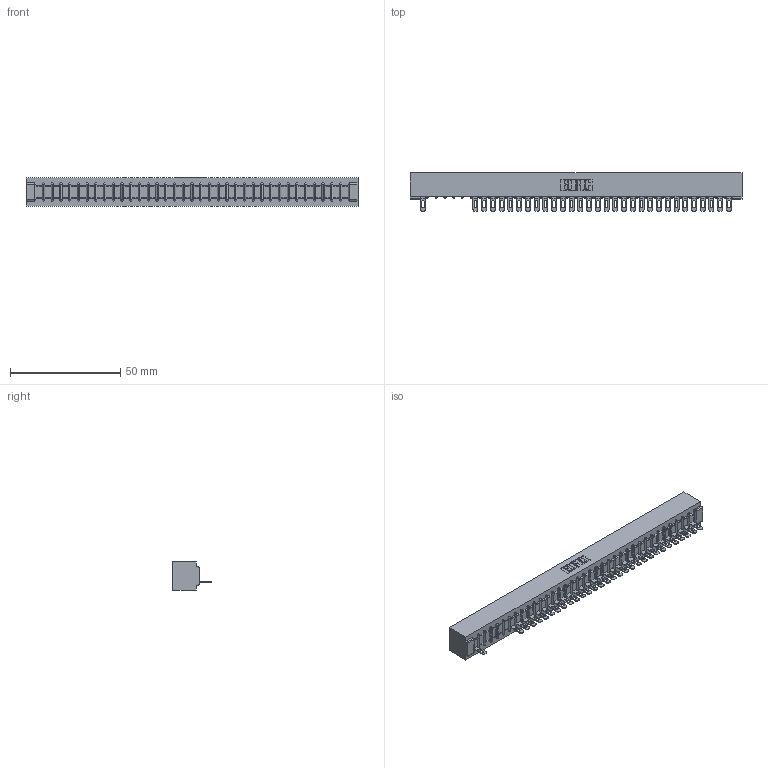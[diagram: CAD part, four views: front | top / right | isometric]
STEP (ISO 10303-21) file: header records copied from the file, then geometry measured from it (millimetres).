
FILE_DESCRIPTION (( 'STEP AP203' ), '1' );
FILE_NAME ('357-036-501-101.STEP', '2018-08-10T05:33:35', ( '' ), ( '' ), 'SwSTEP 2.0', 'SolidWorks 2016', '' );
FILE_SCHEMA (( 'CONFIG_CONTROL_DESIGN' ));
Length unit declared in the file: inch
Products named in the file (3): 307 Part_No Mounting Lugs; 307-290-002_501; 357-036-501-101
Assembly tree (32 placements, depth 2):
  357-036-501-101
    307 Part_No Mounting Lugs
    307-290-002_501  x31
Bounding box: 150.52 x 17.42 x 12.7 mm (x, y, z)
Volume: 16502.9 mm3; surface area: 20251 mm2
Topology: 32 solids, 32 shells, 2603 faces, 7997 edges, 5230 vertices
Faces by surface type: plane 1490, cylinder 1039, sphere 74
Entity records: 31958 total; most frequent: CARTESIAN_POINT 5411, ORIENTED_EDGE 5406, DIRECTION 5257, EDGE_CURVE 2703, VECTOR 2065, LINE 2065, VERTEX_POINT 1750, AXIS2_PLACEMENT_3D 1596
